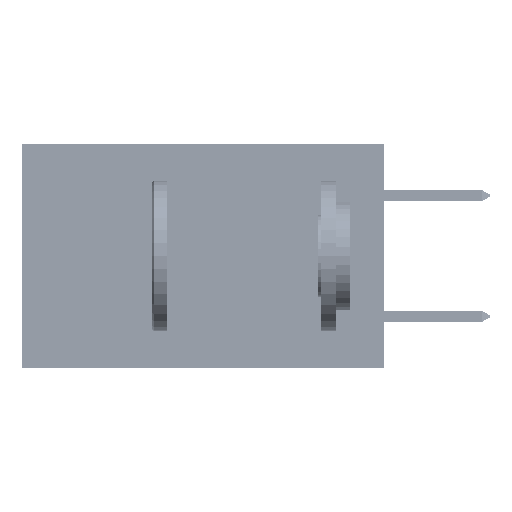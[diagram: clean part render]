
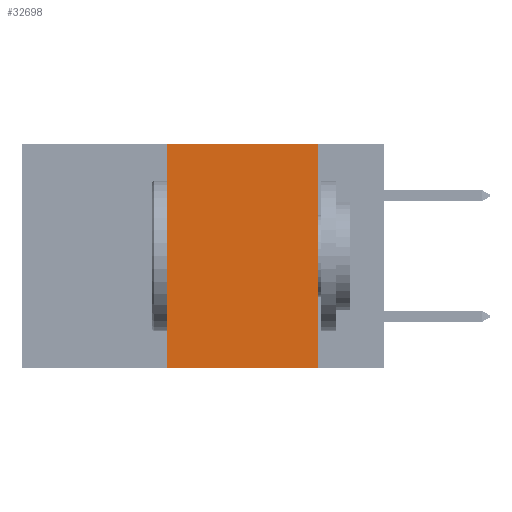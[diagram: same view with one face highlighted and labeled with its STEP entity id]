
A CAD part, left-side view. The second image highlights one B-rep face of the part: STEP entity #32698.
In plain terms, the highlighted planar face has unit normal (-1, 0, 0).
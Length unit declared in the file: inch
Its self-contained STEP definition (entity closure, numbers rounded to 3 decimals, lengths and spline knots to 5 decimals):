
#936 = ORIENTED_EDGE ( 'NONE', *, *, #44685, .F. ) ;
#1260 = CARTESIAN_POINT ( 'NONE',  ( 0., 0.11, 0. ) ) ;
#2521 = LINE ( 'NONE', #15579, #28809 ) ;
#3574 = CARTESIAN_POINT ( 'NONE',  ( 0., 0.6, -0.37 ) ) ;
#9508 = DIRECTION ( 'NONE',  ( 0., 0., -1. ) ) ;
#10082 = CARTESIAN_POINT ( 'NONE',  ( 0., 0.36, 0. ) ) ;
#10921 = ORIENTED_EDGE ( 'NONE', *, *, #21354, .T. ) ;
#11758 = VECTOR ( 'NONE', #30113, 39.37008 ) ;
#11859 = DIRECTION ( 'NONE',  ( 0., 0., -1. ) ) ;
#12905 = LINE ( 'NONE', #37122, #11758 ) ;
#13634 = VERTEX_POINT ( 'NONE', #41182 ) ;
#14350 = AXIS2_PLACEMENT_3D ( 'NONE', #16596, #30963, #9508 ) ;
#15579 = CARTESIAN_POINT ( 'NONE',  ( 0., 0.6, 0. ) ) ;
#15857 = VERTEX_POINT ( 'NONE', #42366 ) ;
#15939 = CARTESIAN_POINT ( 'NONE',  ( 0., 0.11, -0.37 ) ) ;
#16596 = CARTESIAN_POINT ( 'NONE',  ( 0., 0.6, 0. ) ) ;
#20033 = EDGE_CURVE ( 'NONE', #31437, #13634, #2521, .T. ) ;
#21354 = EDGE_CURVE ( 'NONE', #15857, #31236, #30890, .T. ) ;
#21890 = LINE ( 'NONE', #1260, #40888 ) ;
#24922 = EDGE_LOOP ( 'NONE', ( #936, #37232, #27405, #10921 ) ) ;
#27373 = PLANE ( 'NONE',  #14350 ) ;
#27405 = ORIENTED_EDGE ( 'NONE', *, *, #31868, .F. ) ;
#28809 = VECTOR ( 'NONE', #37125, 39.37008 ) ;
#30113 = DIRECTION ( 'NONE',  ( 0., 0., 1. ) ) ;
#30890 = LINE ( 'NONE', #3574, #39264 ) ;
#30963 = DIRECTION ( 'NONE',  ( 1., 0., 0. ) ) ;
#31236 = VERTEX_POINT ( 'NONE', #15939 ) ;
#31437 = VERTEX_POINT ( 'NONE', #10082 ) ;
#31868 = EDGE_CURVE ( 'NONE', #15857, #31437, #12905, .T. ) ;
#32171 = DIRECTION ( 'NONE',  ( 0., -1., 0. ) ) ;
#32698 = ADVANCED_FACE ( 'NONE', ( #37272 ), #27373, .F. ) ;
#37122 = CARTESIAN_POINT ( 'NONE',  ( 0., 0.36, 0. ) ) ;
#37125 = DIRECTION ( 'NONE',  ( 0., -1., 0. ) ) ;
#37232 = ORIENTED_EDGE ( 'NONE', *, *, #20033, .F. ) ;
#37272 = FACE_OUTER_BOUND ( 'NONE', #24922, .T. ) ;
#39264 = VECTOR ( 'NONE', #32171, 39.37008 ) ;
#40888 = VECTOR ( 'NONE', #11859, 39.37008 ) ;
#41182 = CARTESIAN_POINT ( 'NONE',  ( 0., 0.11, 0. ) ) ;
#42366 = CARTESIAN_POINT ( 'NONE',  ( 0., 0.36, -0.37 ) ) ;
#44685 = EDGE_CURVE ( 'NONE', #13634, #31236, #21890, .T. ) ;
